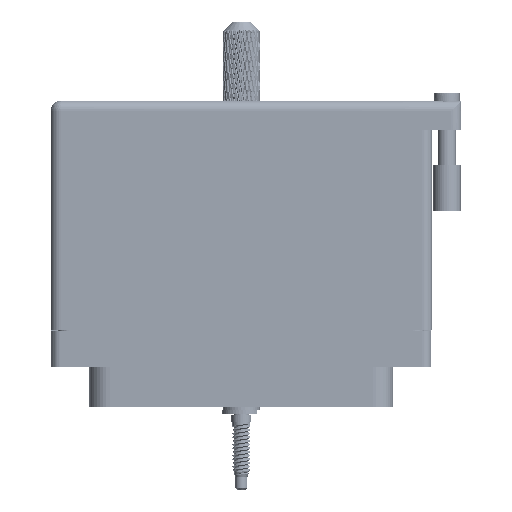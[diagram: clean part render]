
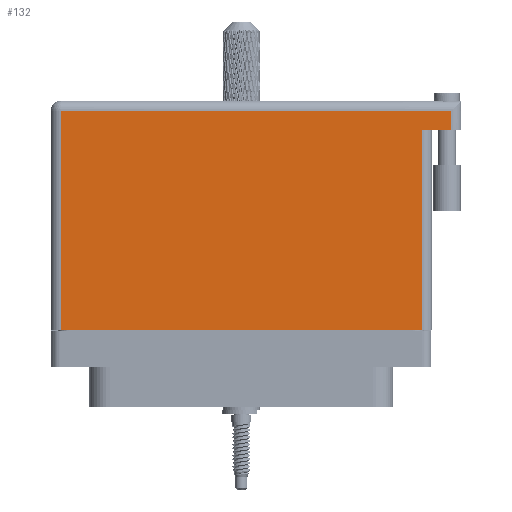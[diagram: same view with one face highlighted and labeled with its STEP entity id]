
A CAD part, front view. The second image highlights one B-rep face of the part: STEP entity #132.
In plain terms, the highlighted face is planar.
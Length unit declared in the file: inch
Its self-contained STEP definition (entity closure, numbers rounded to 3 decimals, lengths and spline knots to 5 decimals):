
#132 = ADVANCED_FACE ( 'NONE', ( #110479 ), #3720, .F. ) ;
#3720 = PLANE ( 'NONE',  #42737 ) ;
#9013 = CARTESIAN_POINT ( 'NONE',  ( -1.23, -0.1, 0.4495 ) ) ;
#9417 = EDGE_CURVE ( 'NONE', #9750, #78221, #100823, .T. ) ;
#9750 = VERTEX_POINT ( 'NONE', #9013 ) ;
#9962 = DIRECTION ( 'NONE',  ( 0., 1., 0. ) ) ;
#14643 = CARTESIAN_POINT ( 'NONE',  ( -1.3, 1.396, 0.4495 ) ) ;
#21653 = EDGE_CURVE ( 'NONE', #78221, #73266, #104290, .T. ) ;
#22412 = DIRECTION ( 'NONE',  ( -1., 0., 0. ) ) ;
#23178 = CARTESIAN_POINT ( 'NONE',  ( 1.43, 1.269, 0.4495 ) ) ;
#23603 = DIRECTION ( 'NONE',  ( -1., 0., 0. ) ) ;
#24614 = VERTEX_POINT ( 'NONE', #117561 ) ;
#24662 = ORIENTED_EDGE ( 'NONE', *, *, #84498, .T. ) ;
#29303 = ORIENTED_EDGE ( 'NONE', *, *, #74357, .F. ) ;
#29335 = LINE ( 'NONE', #33968, #68942 ) ;
#29684 = CARTESIAN_POINT ( 'NONE',  ( 1.23, -0.1, 0.4495 ) ) ;
#33968 = CARTESIAN_POINT ( 'NONE',  ( -1.23, -0.1, 0.4495 ) ) ;
#42737 = AXIS2_PLACEMENT_3D ( 'NONE', #113074, #76992, #22412 ) ;
#44958 = LINE ( 'NONE', #47228, #90256 ) ;
#46997 = VECTOR ( 'NONE', #110640, 39.37008 ) ;
#47228 = CARTESIAN_POINT ( 'NONE',  ( 1.43, 1.466, 0.4495 ) ) ;
#48746 = DIRECTION ( 'NONE',  ( 0., 1., 0. ) ) ;
#52115 = DIRECTION ( 'NONE',  ( 0., -1., 0. ) ) ;
#54057 = VECTOR ( 'NONE', #23603, 39.37008 ) ;
#61816 = ORIENTED_EDGE ( 'NONE', *, *, #9417, .T. ) ;
#68666 = CARTESIAN_POINT ( 'NONE',  ( 1.5, 1.269, 0.4495 ) ) ;
#68942 = VECTOR ( 'NONE', #52115, 39.37008 ) ;
#69458 = VERTEX_POINT ( 'NONE', #23178 ) ;
#71536 = EDGE_LOOP ( 'NONE', ( #61816, #80167, #29303, #24662, #116207, #77995 ) ) ;
#73266 = VERTEX_POINT ( 'NONE', #113626 ) ;
#74357 = EDGE_CURVE ( 'NONE', #69458, #73266, #86655, .T. ) ;
#76992 = DIRECTION ( 'NONE',  ( 0., 0., -1. ) ) ;
#77995 = ORIENTED_EDGE ( 'NONE', *, *, #85002, .T. ) ;
#78221 = VERTEX_POINT ( 'NONE', #29684 ) ;
#80167 = ORIENTED_EDGE ( 'NONE', *, *, #21653, .T. ) ;
#82663 = EDGE_CURVE ( 'NONE', #96805, #24614, #103901, .T. ) ;
#84498 = EDGE_CURVE ( 'NONE', #69458, #96805, #44958, .T. ) ;
#85002 = EDGE_CURVE ( 'NONE', #24614, #9750, #29335, .T. ) ;
#86655 = LINE ( 'NONE', #68666, #54057 ) ;
#90256 = VECTOR ( 'NONE', #48746, 39.37008 ) ;
#94623 = CARTESIAN_POINT ( 'NONE',  ( 1.43, 1.396, 0.4495 ) ) ;
#96805 = VERTEX_POINT ( 'NONE', #94623 ) ;
#97735 = CARTESIAN_POINT ( 'NONE',  ( 1.23, 1.269, 0.4495 ) ) ;
#98170 = VECTOR ( 'NONE', #114800, 39.37008 ) ;
#100823 = LINE ( 'NONE', #101078, #46997 ) ;
#101078 = CARTESIAN_POINT ( 'NONE',  ( -1.3, -0.1, 0.4495 ) ) ;
#103901 = LINE ( 'NONE', #14643, #98170 ) ;
#104290 = LINE ( 'NONE', #97735, #109851 ) ;
#109851 = VECTOR ( 'NONE', #9962, 39.37008 ) ;
#110479 = FACE_OUTER_BOUND ( 'NONE', #71536, .T. ) ;
#110640 = DIRECTION ( 'NONE',  ( 1., 0., 0. ) ) ;
#113074 = CARTESIAN_POINT ( 'NONE',  ( -1.3, 1.466, 0.4495 ) ) ;
#113626 = CARTESIAN_POINT ( 'NONE',  ( 1.23, 1.269, 0.4495 ) ) ;
#114800 = DIRECTION ( 'NONE',  ( -1., 0., 0. ) ) ;
#116207 = ORIENTED_EDGE ( 'NONE', *, *, #82663, .T. ) ;
#117561 = CARTESIAN_POINT ( 'NONE',  ( -1.23, 1.396, 0.4495 ) ) ;
